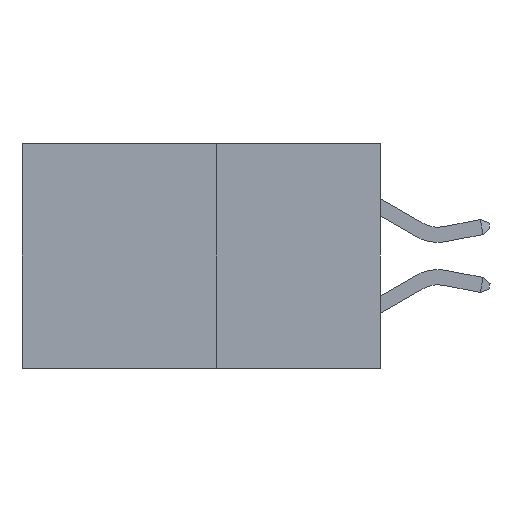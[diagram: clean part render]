
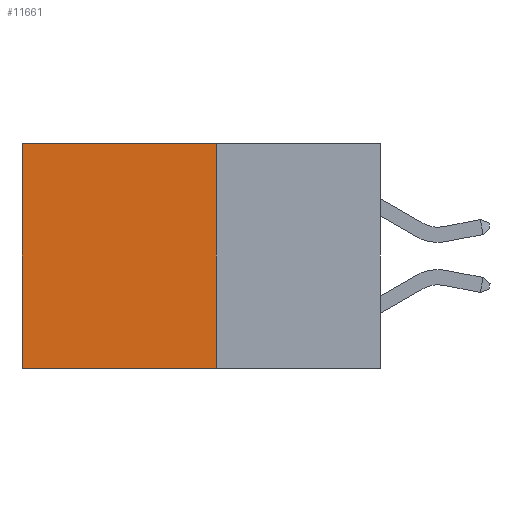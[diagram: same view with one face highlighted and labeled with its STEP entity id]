
A CAD part, left-side view. The second image highlights one B-rep face of the part: STEP entity #11661.
In plain terms, the highlighted planar face has unit normal (-1, 0, 0).
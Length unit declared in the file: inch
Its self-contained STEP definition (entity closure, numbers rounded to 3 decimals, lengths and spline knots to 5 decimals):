
#100 = CARTESIAN_POINT ( 'NONE',  ( 0.277, 0.59, -0.37 ) ) ;
#595 = DIRECTION ( 'NONE',  ( 0., 0., -1. ) ) ;
#1334 = DIRECTION ( 'NONE',  ( 0., 0., -1. ) ) ;
#1873 = EDGE_LOOP ( 'NONE', ( #8958, #8985, #12881, #6035 ) ) ;
#2615 = AXIS2_PLACEMENT_3D ( 'NONE', #4987, #8797, #1334 ) ;
#3399 = LINE ( 'NONE', #8090, #6715 ) ;
#3570 = EDGE_CURVE ( 'NONE', #7485, #4494, #3922, .T. ) ;
#3800 = EDGE_CURVE ( 'NONE', #11963, #7485, #10649, .T. ) ;
#3922 = LINE ( 'NONE', #14204, #12947 ) ;
#4494 = VERTEX_POINT ( 'NONE', #100 ) ;
#4987 = CARTESIAN_POINT ( 'NONE',  ( 0.277, 0.27, -0.37 ) ) ;
#5561 = CARTESIAN_POINT ( 'NONE',  ( 0.277, 0.27, -0.37 ) ) ;
#6035 = ORIENTED_EDGE ( 'NONE', *, *, #9794, .T. ) ;
#6220 = DIRECTION ( 'NONE',  ( 0., 0., -1. ) ) ;
#6569 = CARTESIAN_POINT ( 'NONE',  ( 0.277, 0.59, 0. ) ) ;
#6715 = VECTOR ( 'NONE', #595, 39.37008 ) ;
#6839 = CARTESIAN_POINT ( 'NONE',  ( 0.277, 0.27, 0. ) ) ;
#6889 = VECTOR ( 'NONE', #9714, 39.37008 ) ;
#7485 = VERTEX_POINT ( 'NONE', #8862 ) ;
#8036 = DIRECTION ( 'NONE',  ( 0., 1., 0. ) ) ;
#8090 = CARTESIAN_POINT ( 'NONE',  ( 0.277, 0.59, -0.37 ) ) ;
#8797 = DIRECTION ( 'NONE',  ( 1., 0., 0. ) ) ;
#8862 = CARTESIAN_POINT ( 'NONE',  ( 0.277, 0.27, -0.37 ) ) ;
#8958 = ORIENTED_EDGE ( 'NONE', *, *, #15180, .T. ) ;
#8985 = ORIENTED_EDGE ( 'NONE', *, *, #3570, .F. ) ;
#9683 = CARTESIAN_POINT ( 'NONE',  ( 0.277, 0.27, 0. ) ) ;
#9712 = FACE_OUTER_BOUND ( 'NONE', #1873, .T. ) ;
#9714 = DIRECTION ( 'NONE',  ( 0., 1., 0. ) ) ;
#9794 = EDGE_CURVE ( 'NONE', #11963, #15721, #10134, .T. ) ;
#9911 = VECTOR ( 'NONE', #6220, 39.37008 ) ;
#10134 = LINE ( 'NONE', #9683, #6889 ) ;
#10649 = LINE ( 'NONE', #5561, #9911 ) ;
#11661 = ADVANCED_FACE ( 'NONE', ( #9712 ), #14796, .F. ) ;
#11963 = VERTEX_POINT ( 'NONE', #6839 ) ;
#12881 = ORIENTED_EDGE ( 'NONE', *, *, #3800, .F. ) ;
#12947 = VECTOR ( 'NONE', #8036, 39.37008 ) ;
#14204 = CARTESIAN_POINT ( 'NONE',  ( 0.277, 0.27, -0.37 ) ) ;
#14796 = PLANE ( 'NONE',  #2615 ) ;
#15180 = EDGE_CURVE ( 'NONE', #15721, #4494, #3399, .T. ) ;
#15721 = VERTEX_POINT ( 'NONE', #6569 ) ;
